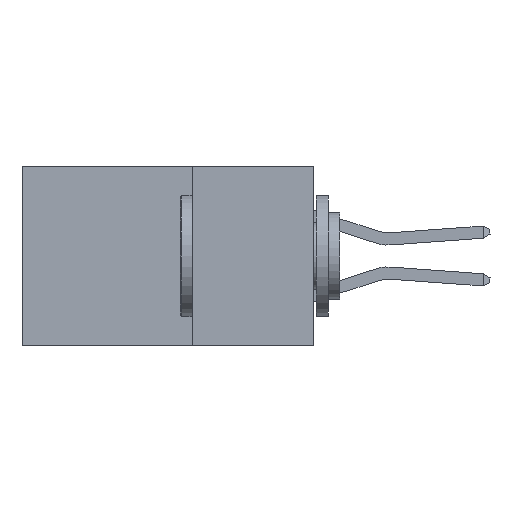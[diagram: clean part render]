
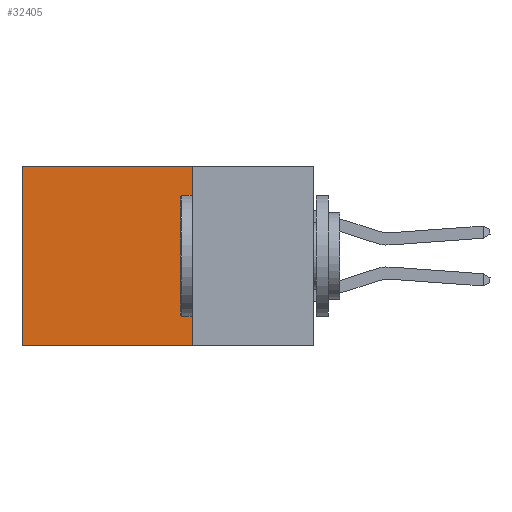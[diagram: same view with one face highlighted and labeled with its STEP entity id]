
A CAD part, left-side view. The second image highlights one B-rep face of the part: STEP entity #32405.
In plain terms, the highlighted planar face has unit normal (-1, 0, 0).
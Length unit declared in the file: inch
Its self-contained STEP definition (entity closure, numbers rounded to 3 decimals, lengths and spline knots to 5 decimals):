
#87 = LINE ( 'NONE', #23529, #19852 ) ;
#432 = VECTOR ( 'NONE', #17968, 39.37008 ) ;
#531 = VERTEX_POINT ( 'NONE', #28897 ) ;
#1441 = ORIENTED_EDGE ( 'NONE', *, *, #27413, .T. ) ;
#2099 = VERTEX_POINT ( 'NONE', #11469 ) ;
#5169 = CARTESIAN_POINT ( 'NONE',  ( 0.2875, 0.25, 0. ) ) ;
#5666 = ORIENTED_EDGE ( 'NONE', *, *, #31651, .F. ) ;
#7613 = AXIS2_PLACEMENT_3D ( 'NONE', #23633, #7891, #11155 ) ;
#7891 = DIRECTION ( 'NONE',  ( 1., 0., 0. ) ) ;
#9128 = ORIENTED_EDGE ( 'NONE', *, *, #39902, .F. ) ;
#11155 = DIRECTION ( 'NONE',  ( 0., 0., -1. ) ) ;
#11469 = CARTESIAN_POINT ( 'NONE',  ( 0.2875, 0.6, 0. ) ) ;
#17517 = PLANE ( 'NONE',  #7613 ) ;
#17968 = DIRECTION ( 'NONE',  ( 0., 1., 0. ) ) ;
#19852 = VECTOR ( 'NONE', #26719, 39.37008 ) ;
#20184 = LINE ( 'NONE', #36884, #432 ) ;
#20571 = CARTESIAN_POINT ( 'NONE',  ( 0.2875, 0.25, -0.37 ) ) ;
#21488 = DIRECTION ( 'NONE',  ( 0., 1., 0. ) ) ;
#23529 = CARTESIAN_POINT ( 'NONE',  ( 0.2875, 0.25, 0. ) ) ;
#23633 = CARTESIAN_POINT ( 'NONE',  ( 0.2875, 0.25, 0. ) ) ;
#26719 = DIRECTION ( 'NONE',  ( 0., 0., -1. ) ) ;
#27413 = EDGE_CURVE ( 'NONE', #2099, #531, #40376, .T. ) ;
#28897 = CARTESIAN_POINT ( 'NONE',  ( 0.2875, 0.6, -0.37 ) ) ;
#29168 = VECTOR ( 'NONE', #33040, 39.37008 ) ;
#30725 = LINE ( 'NONE', #40372, #37683 ) ;
#31651 = EDGE_CURVE ( 'NONE', #33701, #36009, #87, .T. ) ;
#31755 = EDGE_LOOP ( 'NONE', ( #1441, #9128, #5666, #36331 ) ) ;
#32121 = FACE_OUTER_BOUND ( 'NONE', #31755, .T. ) ;
#32405 = ADVANCED_FACE ( 'NONE', ( #32121 ), #17517, .F. ) ;
#33040 = DIRECTION ( 'NONE',  ( 0., 0., -1. ) ) ;
#33701 = VERTEX_POINT ( 'NONE', #5169 ) ;
#36009 = VERTEX_POINT ( 'NONE', #20571 ) ;
#36074 = CARTESIAN_POINT ( 'NONE',  ( 0.2875, 0.6, 0. ) ) ;
#36331 = ORIENTED_EDGE ( 'NONE', *, *, #37501, .T. ) ;
#36884 = CARTESIAN_POINT ( 'NONE',  ( 0.2875, 0.25, -0.37 ) ) ;
#37501 = EDGE_CURVE ( 'NONE', #33701, #2099, #30725, .T. ) ;
#37683 = VECTOR ( 'NONE', #21488, 39.37008 ) ;
#39902 = EDGE_CURVE ( 'NONE', #36009, #531, #20184, .T. ) ;
#40372 = CARTESIAN_POINT ( 'NONE',  ( 0.2875, 0.25, 0. ) ) ;
#40376 = LINE ( 'NONE', #36074, #29168 ) ;
